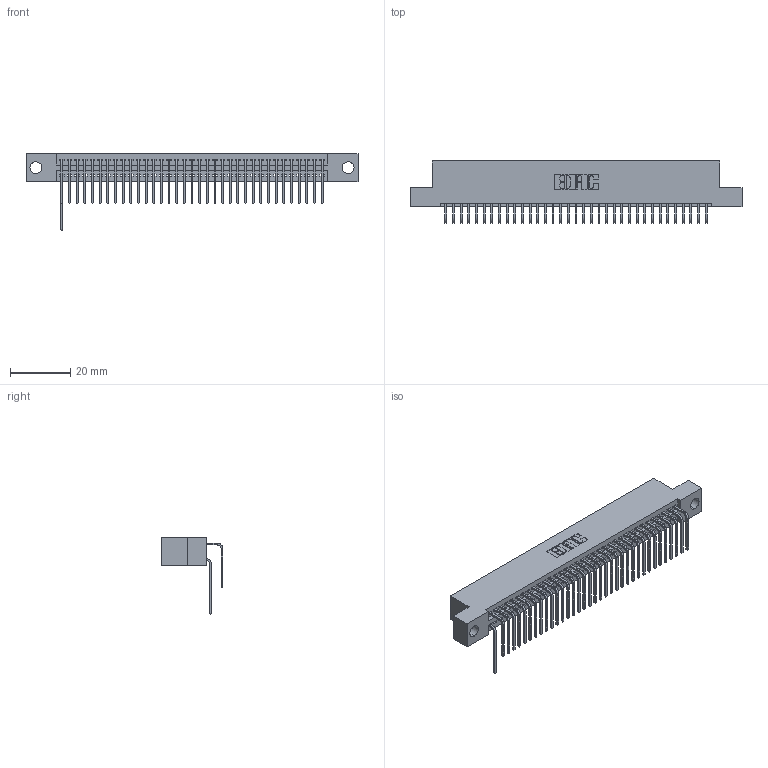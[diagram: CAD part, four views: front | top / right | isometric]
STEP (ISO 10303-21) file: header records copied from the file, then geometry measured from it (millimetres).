
FILE_DESCRIPTION (( 'STEP AP203' ), '1' );
FILE_NAME ('395-070-559-204.STEP', '2018-11-27T02:55:37', ( '' ), ( '' ), 'SwSTEP 2.0', 'SolidWorks 2016', '' );
FILE_SCHEMA (( 'CONFIG_CONTROL_DESIGN' ));
Length unit declared in the file: inch
Products named in the file (4): 345-292-001_559 Tail - 2; 345-292-001_558 559 Tail - 1; 345 Part_Flush Mounting Lugs - 0.156 Dia-TH; 395-070-559-204
Assembly tree (37 placements, depth 2):
  395-070-559-204
    345 Part_Flush Mounting Lugs - 0.156 Dia-TH
    345-292-001_558 559 Tail - 1
    345-292-001_559 Tail - 2  x35
Bounding box: 110.11 x 20.56 x 25.53 mm (x, y, z)
Volume: 10444.5 mm3; surface area: 14359 mm2
Topology: 37 solids, 37 shells, 2270 faces, 6839 edges, 4510 vertices
Faces by surface type: plane 1578, cylinder 692
Entity records: 28971 total; most frequent: CARTESIAN_POINT 5057, ORIENTED_EDGE 4974, DIRECTION 4403, EDGE_CURVE 2487, VECTOR 2175, LINE 2175, VERTEX_POINT 1654, AXIS2_PLACEMENT_3D 1114
